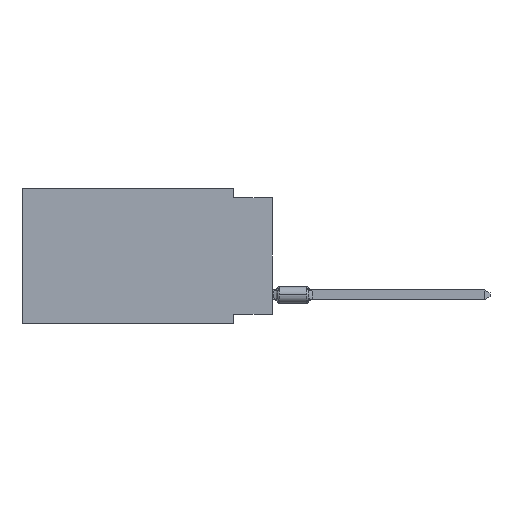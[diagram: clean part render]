
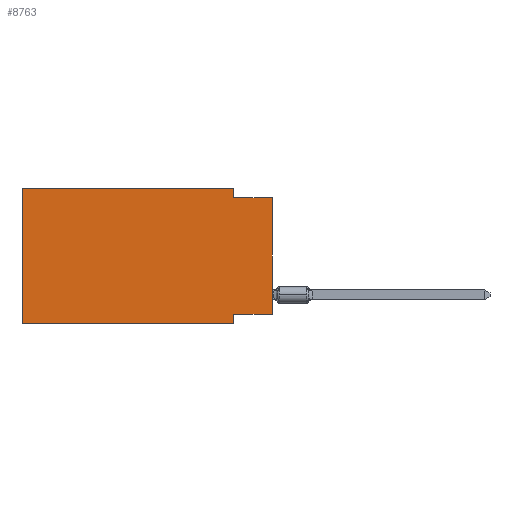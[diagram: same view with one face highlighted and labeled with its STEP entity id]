
A CAD part, left-side view. The second image highlights one B-rep face of the part: STEP entity #8763.
In plain terms, the highlighted planar face has unit normal (-1, 0, 0).
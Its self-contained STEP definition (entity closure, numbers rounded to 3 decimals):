
#20 = EDGE_CURVE ( 'NONE', #11036, #7879, #11348, .T. ) ;
#63 = VECTOR ( 'NONE', #4443, 1000. ) ;
#295 = CARTESIAN_POINT ( 'NONE',  ( 0., 16.383, -8.89 ) ) ;
#297 = VERTEX_POINT ( 'NONE', #2179 ) ;
#475 = LINE ( 'NONE', #12215, #944 ) ;
#492 = VERTEX_POINT ( 'NONE', #9641 ) ;
#944 = VECTOR ( 'NONE', #4698, 1000. ) ;
#1294 = CARTESIAN_POINT ( 'NONE',  ( 0., 16.383, -8.89 ) ) ;
#1454 = ORIENTED_EDGE ( 'NONE', *, *, #3357, .F. ) ;
#1728 = DIRECTION ( 'NONE',  ( 0., 1., 0. ) ) ;
#1799 = VERTEX_POINT ( 'NONE', #2457 ) ;
#1875 = ORIENTED_EDGE ( 'NONE', *, *, #12661, .F. ) ;
#2017 = EDGE_CURVE ( 'NONE', #5069, #1799, #9167, .T. ) ;
#2045 = ORIENTED_EDGE ( 'NONE', *, *, #12402, .T. ) ;
#2179 = CARTESIAN_POINT ( 'NONE',  ( 0., 2.54, -8.89 ) ) ;
#2275 = ORIENTED_EDGE ( 'NONE', *, *, #4685, .F. ) ;
#2457 = CARTESIAN_POINT ( 'NONE',  ( 0., 16.383, 0. ) ) ;
#2531 = CARTESIAN_POINT ( 'NONE',  ( 0., 0., -0.635 ) ) ;
#3124 = DIRECTION ( 'NONE',  ( 0., 0., 1. ) ) ;
#3237 = CARTESIAN_POINT ( 'NONE',  ( 0., 2.54, -8.89 ) ) ;
#3357 = EDGE_CURVE ( 'NONE', #11959, #8928, #11102, .T. ) ;
#3409 = CARTESIAN_POINT ( 'NONE',  ( 0., 2.54, -8.255 ) ) ;
#3732 = VECTOR ( 'NONE', #8639, 1000. ) ;
#3979 = VECTOR ( 'NONE', #4326, 1000. ) ;
#4229 = CARTESIAN_POINT ( 'NONE',  ( 0., 16.383, 0. ) ) ;
#4297 = DIRECTION ( 'NONE',  ( 0., 0., -1. ) ) ;
#4326 = DIRECTION ( 'NONE',  ( 0., 0., -1. ) ) ;
#4343 = CARTESIAN_POINT ( 'NONE',  ( 0., 16.383, 0. ) ) ;
#4443 = DIRECTION ( 'NONE',  ( 0., -1., 0. ) ) ;
#4685 = EDGE_CURVE ( 'NONE', #7879, #492, #11841, .T. ) ;
#4698 = DIRECTION ( 'NONE',  ( 0., 0., 1. ) ) ;
#5022 = ORIENTED_EDGE ( 'NONE', *, *, #2017, .F. ) ;
#5069 = VERTEX_POINT ( 'NONE', #1294 ) ;
#5104 = CARTESIAN_POINT ( 'NONE',  ( 0., 2.54, 0. ) ) ;
#5124 = FACE_OUTER_BOUND ( 'NONE', #6912, .T. ) ;
#5823 = VECTOR ( 'NONE', #8343, 1000. ) ;
#6268 = VECTOR ( 'NONE', #8748, 1000. ) ;
#6513 = LINE ( 'NONE', #4343, #6268 ) ;
#6912 = EDGE_LOOP ( 'NONE', ( #2045, #2275, #9749, #9463, #5022, #7550, #1875, #1454 ) ) ;
#7550 = ORIENTED_EDGE ( 'NONE', *, *, #11905, .T. ) ;
#7879 = VERTEX_POINT ( 'NONE', #9850 ) ;
#8293 = DIRECTION ( 'NONE',  ( 1., 0., 0. ) ) ;
#8343 = DIRECTION ( 'NONE',  ( 0., 0., -1. ) ) ;
#8639 = DIRECTION ( 'NONE',  ( 0., -1., 0. ) ) ;
#8748 = DIRECTION ( 'NONE',  ( 0., -1., 0. ) ) ;
#8763 = ADVANCED_FACE ( 'NONE', ( #5124 ), #11369, .F. ) ;
#8928 = VERTEX_POINT ( 'NONE', #3409 ) ;
#9167 = LINE ( 'NONE', #11485, #12546 ) ;
#9324 = EDGE_CURVE ( 'NONE', #1799, #11036, #6513, .T. ) ;
#9463 = ORIENTED_EDGE ( 'NONE', *, *, #9324, .F. ) ;
#9641 = CARTESIAN_POINT ( 'NONE',  ( 0., 0., -0.635 ) ) ;
#9749 = ORIENTED_EDGE ( 'NONE', *, *, #20, .F. ) ;
#9850 = CARTESIAN_POINT ( 'NONE',  ( 0., 2.54, -0.635 ) ) ;
#9874 = CARTESIAN_POINT ( 'NONE',  ( 0., 0., -8.255 ) ) ;
#11036 = VERTEX_POINT ( 'NONE', #11344 ) ;
#11102 = LINE ( 'NONE', #9874, #11761 ) ;
#11344 = CARTESIAN_POINT ( 'NONE',  ( 0., 2.54, 0. ) ) ;
#11348 = LINE ( 'NONE', #5104, #5823 ) ;
#11369 = PLANE ( 'NONE',  #12779 ) ;
#11485 = CARTESIAN_POINT ( 'NONE',  ( 0., 16.383, 0. ) ) ;
#11530 = LINE ( 'NONE', #3237, #3979 ) ;
#11761 = VECTOR ( 'NONE', #1728, 1000. ) ;
#11841 = LINE ( 'NONE', #2531, #3732 ) ;
#11905 = EDGE_CURVE ( 'NONE', #5069, #297, #12744, .T. ) ;
#11959 = VERTEX_POINT ( 'NONE', #13076 ) ;
#12215 = CARTESIAN_POINT ( 'NONE',  ( 0., 0., 0. ) ) ;
#12402 = EDGE_CURVE ( 'NONE', #11959, #492, #475, .T. ) ;
#12546 = VECTOR ( 'NONE', #3124, 1000. ) ;
#12661 = EDGE_CURVE ( 'NONE', #8928, #297, #11530, .T. ) ;
#12744 = LINE ( 'NONE', #295, #63 ) ;
#12779 = AXIS2_PLACEMENT_3D ( 'NONE', #4229, #8293, #4297 ) ;
#13076 = CARTESIAN_POINT ( 'NONE',  ( 0., 0., -8.255 ) ) ;
